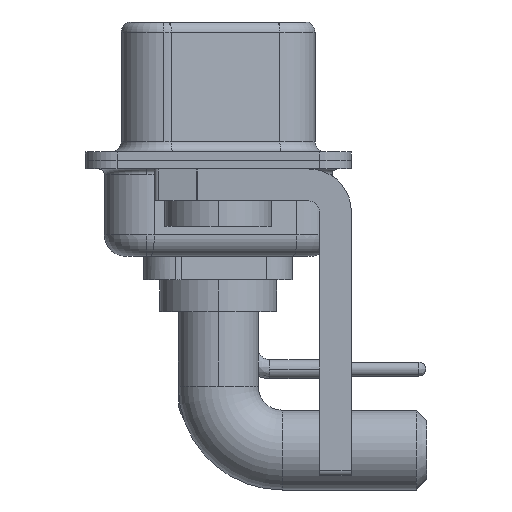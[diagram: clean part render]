
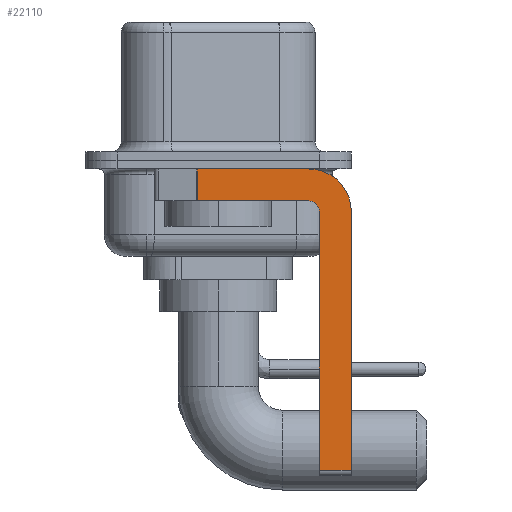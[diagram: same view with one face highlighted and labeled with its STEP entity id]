
A CAD part, left-side view. The second image highlights one B-rep face of the part: STEP entity #22110.
In plain terms, the highlighted planar face has unit normal (-1, 0, 0).
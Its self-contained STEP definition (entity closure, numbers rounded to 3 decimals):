
#516 = CARTESIAN_POINT ( 'NONE',  ( -2.9, 3., -0.4 ) ) ;
#780 = CARTESIAN_POINT ( 'NONE',  ( -2.9, -6.25, -14.55 ) ) ;
#793 = VERTEX_POINT ( 'NONE', #23980 ) ;
#906 = LINE ( 'NONE', #10027, #25408 ) ;
#1059 = ORIENTED_EDGE ( 'NONE', *, *, #17287, .F. ) ;
#1637 = EDGE_LOOP ( 'NONE', ( #24927, #8968, #8106, #18273, #28127, #3579, #1059, #9177 ) ) ;
#2906 = LINE ( 'NONE', #14707, #9532 ) ;
#3204 = CARTESIAN_POINT ( 'NONE',  ( -2.9, -4.75, -14.8 ) ) ;
#3313 = VERTEX_POINT ( 'NONE', #27633 ) ;
#3327 = AXIS2_PLACEMENT_3D ( 'NONE', #7897, #16730, #18954 ) ;
#3497 = CARTESIAN_POINT ( 'NONE',  ( -2.9, -4.25, -2.4 ) ) ;
#3499 = VERTEX_POINT ( 'NONE', #780 ) ;
#3579 = ORIENTED_EDGE ( 'NONE', *, *, #15518, .T. ) ;
#3959 = LINE ( 'NONE', #28998, #9958 ) ;
#4626 = CARTESIAN_POINT ( 'NONE',  ( -2.9, -6.25, -2.4 ) ) ;
#5386 = EDGE_CURVE ( 'NONE', #23751, #7080, #906, .T. ) ;
#5646 = VERTEX_POINT ( 'NONE', #4626 ) ;
#5749 = CARTESIAN_POINT ( 'NONE',  ( -2.9, 0.978, -0.4 ) ) ;
#5849 = CARTESIAN_POINT ( 'NONE',  ( -2.9, -4.75, -14.55 ) ) ;
#6346 = VECTOR ( 'NONE', #16346, 1000. ) ;
#7080 = VERTEX_POINT ( 'NONE', #9086 ) ;
#7140 = VECTOR ( 'NONE', #10218, 1000. ) ;
#7897 = CARTESIAN_POINT ( 'NONE',  ( -2.9, -4.25, -2.4 ) ) ;
#8106 = ORIENTED_EDGE ( 'NONE', *, *, #5386, .F. ) ;
#8968 = ORIENTED_EDGE ( 'NONE', *, *, #16273, .T. ) ;
#9086 = CARTESIAN_POINT ( 'NONE',  ( -2.9, 0.978, -1.9 ) ) ;
#9177 = ORIENTED_EDGE ( 'NONE', *, *, #26895, .F. ) ;
#9532 = VECTOR ( 'NONE', #28111, 1000. ) ;
#9540 = CARTESIAN_POINT ( 'NONE',  ( -2.9, -4.25, -14.55 ) ) ;
#9958 = VECTOR ( 'NONE', #12767, 1000. ) ;
#10027 = CARTESIAN_POINT ( 'NONE',  ( -2.9, -4.25, -1.9 ) ) ;
#10218 = DIRECTION ( 'NONE',  ( 0., -1., 0. ) ) ;
#11621 = CIRCLE ( 'NONE', #15887, 2. ) ;
#11631 = LINE ( 'NONE', #9540, #23720 ) ;
#11928 = AXIS2_PLACEMENT_3D ( 'NONE', #20561, #29494, #29343 ) ;
#12172 = VERTEX_POINT ( 'NONE', #5849 ) ;
#12767 = DIRECTION ( 'NONE',  ( 0., 0., -1. ) ) ;
#13106 = PLANE ( 'NONE',  #11928 ) ;
#14707 = CARTESIAN_POINT ( 'NONE',  ( -2.9, -6.25, -2.4 ) ) ;
#15518 = EDGE_CURVE ( 'NONE', #12172, #3499, #11631, .T. ) ;
#15609 = CARTESIAN_POINT ( 'NONE',  ( -2.9, -4.25, -1.9 ) ) ;
#15887 = AXIS2_PLACEMENT_3D ( 'NONE', #3497, #22096, #26843 ) ;
#16273 = EDGE_CURVE ( 'NONE', #24050, #7080, #3959, .T. ) ;
#16346 = DIRECTION ( 'NONE',  ( 0., 0., 1. ) ) ;
#16730 = DIRECTION ( 'NONE',  ( -1., 0., 0. ) ) ;
#17214 = EDGE_CURVE ( 'NONE', #24050, #793, #28398, .T. ) ;
#17287 = EDGE_CURVE ( 'NONE', #5646, #3499, #2906, .T. ) ;
#18273 = ORIENTED_EDGE ( 'NONE', *, *, #21843, .F. ) ;
#18954 = DIRECTION ( 'NONE',  ( 0., 0., 1. ) ) ;
#20561 = CARTESIAN_POINT ( 'NONE',  ( -2.9, -4.25, -2.4 ) ) ;
#21843 = EDGE_CURVE ( 'NONE', #3313, #23751, #22379, .T. ) ;
#22096 = DIRECTION ( 'NONE',  ( 1., 0., 0. ) ) ;
#22110 = ADVANCED_FACE ( 'NONE', ( #24420 ), #13106, .F. ) ;
#22379 = CIRCLE ( 'NONE', #3327, 0.5 ) ;
#23401 = DIRECTION ( 'NONE',  ( 0., -1., 0. ) ) ;
#23720 = VECTOR ( 'NONE', #23401, 1000. ) ;
#23751 = VERTEX_POINT ( 'NONE', #15609 ) ;
#23980 = CARTESIAN_POINT ( 'NONE',  ( -2.9, -4.25, -0.4 ) ) ;
#24050 = VERTEX_POINT ( 'NONE', #5749 ) ;
#24420 = FACE_OUTER_BOUND ( 'NONE', #1637, .T. ) ;
#24927 = ORIENTED_EDGE ( 'NONE', *, *, #17214, .F. ) ;
#25408 = VECTOR ( 'NONE', #28207, 1000. ) ;
#25713 = LINE ( 'NONE', #3204, #6346 ) ;
#26741 = EDGE_CURVE ( 'NONE', #12172, #3313, #25713, .T. ) ;
#26843 = DIRECTION ( 'NONE',  ( 0., 0., -1. ) ) ;
#26895 = EDGE_CURVE ( 'NONE', #793, #5646, #11621, .T. ) ;
#27633 = CARTESIAN_POINT ( 'NONE',  ( -2.9, -4.75, -2.4 ) ) ;
#28111 = DIRECTION ( 'NONE',  ( 0., 0., -1. ) ) ;
#28127 = ORIENTED_EDGE ( 'NONE', *, *, #26741, .F. ) ;
#28207 = DIRECTION ( 'NONE',  ( 0., 1., 0. ) ) ;
#28398 = LINE ( 'NONE', #516, #7140 ) ;
#28998 = CARTESIAN_POINT ( 'NONE',  ( -2.9, 0.978, -1.9 ) ) ;
#29343 = DIRECTION ( 'NONE',  ( 0., 0., -1. ) ) ;
#29494 = DIRECTION ( 'NONE',  ( 1., 0., 0. ) ) ;
